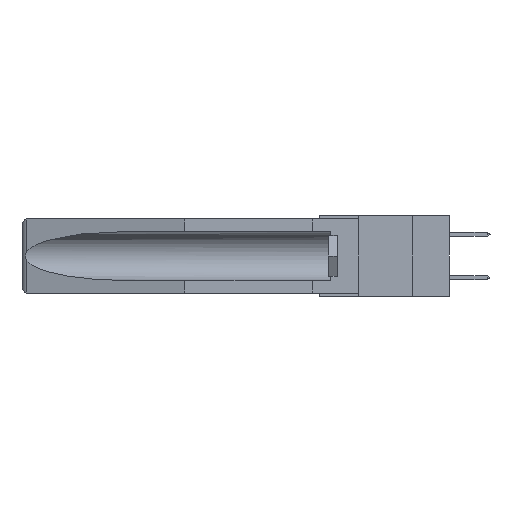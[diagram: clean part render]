
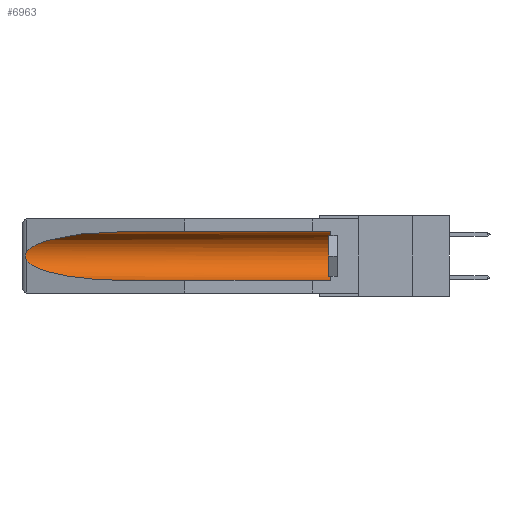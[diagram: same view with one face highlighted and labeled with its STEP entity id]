
A CAD part, left-side view. The second image highlights one B-rep face of the part: STEP entity #6963.
In plain terms, the highlighted cylindrical face has radius 2.857 mm (diameter 5.715 mm), a partial arc.
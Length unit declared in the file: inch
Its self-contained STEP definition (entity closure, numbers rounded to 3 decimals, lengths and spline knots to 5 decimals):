
#59 = VERTEX_POINT ( 'NONE', #10815 ) ;
#134 = DIRECTION ( 'NONE',  ( 0., 1., 0. ) ) ;
#174 = DIRECTION ( 'NONE',  ( 0., 1., 0. ) ) ;
#316 = FACE_OUTER_BOUND ( 'NONE', #22766, .T. ) ;
#932 = DIRECTION ( 'NONE',  ( 0., 0., 1. ) ) ;
#1498 = VERTEX_POINT ( 'NONE', #21890 ) ;
#1548 = CIRCLE ( 'NONE', #16449, 0.1125 ) ;
#3042 = LINE ( 'NONE', #25327, #4693 ) ;
#3285 = CARTESIAN_POINT ( 'NONE',  ( 0.26655, 1.53094, -0.18657 ) ) ;
#3318 = CARTESIAN_POINT ( 'NONE',  ( 0.25451, 1.48313, -0.24835 ) ) ;
#4693 = VECTOR ( 'NONE', #9252, 39.37008 ) ;
#4978 = CARTESIAN_POINT ( 'NONE',  ( 0.25451, 1.48313, -0.09465 ) ) ;
#6385 = DIRECTION ( 'NONE',  ( 0., -1., 0. ) ) ;
#6556 = CARTESIAN_POINT ( 'NONE',  ( 0.155, 1.07973, -0.284 ) ) ;
#6676 = AXIS2_PLACEMENT_3D ( 'NONE', #10290, #134, #32655 ) ;
#6963 = ADVANCED_FACE ( 'NONE', ( #316 ), #26231, .F. ) ;
#7636 = CARTESIAN_POINT ( 'NONE',  ( 0.26537, 1.52718, -0.14972 ) ) ;
#8374 = CARTESIAN_POINT ( 'NONE',  ( 0.2673, 1.53269, -0.17917 ) ) ;
#8610 = CARTESIAN_POINT ( 'NONE',  ( 0.26597, 1.5296, -0.19026 ) ) ;
#9143 = ORIENTED_EDGE ( 'NONE', *, *, #29280, .T. ) ;
#9252 = DIRECTION ( 'NONE',  ( 0., 1., 0. ) ) ;
#10238 = CARTESIAN_POINT ( 'NONE',  ( 0.21114, 1.30732, -0.059 ) ) ;
#10290 = CARTESIAN_POINT ( 'NONE',  ( 0.155, -0.30754, -0.1715 ) ) ;
#10815 = CARTESIAN_POINT ( 'NONE',  ( 0.26537, 1.52718, -0.14972 ) ) ;
#11395 = CARTESIAN_POINT ( 'NONE',  ( 0.155, 0.126, -0.059 ) ) ;
#11429 = CARTESIAN_POINT ( 'NONE',  ( 0.2675, 1.53308, -0.16763 ) ) ;
#11684 = CARTESIAN_POINT ( 'NONE',  ( 0.155, 1.07973, -0.284 ) ) ;
#13433 = ORIENTED_EDGE ( 'NONE', *, *, #33582, .T. ) ;
#15257 = EDGE_CURVE ( 'NONE', #30321, #20262, #20143, .T. ) ;
#15938 = CARTESIAN_POINT ( 'NONE',  ( 0.155, 0.126, -0.284 ) ) ;
#16397 = CARTESIAN_POINT ( 'NONE',  ( 0.26597, 1.52961, -0.15275 ) ) ;
#16449 = AXIS2_PLACEMENT_3D ( 'NONE', #19545, #6385, #932 ) ;
#16843 = CARTESIAN_POINT ( 'NONE',  ( 0.26654, 1.53092, -0.15636 ) ) ;
#18236 = CARTESIAN_POINT ( 'NONE',  ( 0.155, 1.07973, -0.059 ) ) ;
#19545 = CARTESIAN_POINT ( 'NONE',  ( 0.155, 0.126, -0.1715 ) ) ;
#20061 =( BOUNDED_CURVE ( )  B_SPLINE_CURVE ( 3, ( #27736, #3318, #29985, #11684 ),
 .UNSPECIFIED., .F., .F. ) 
 B_SPLINE_CURVE_WITH_KNOTS ( ( 4, 4 ),
 ( 0.1948, 1.5708 ),
 .UNSPECIFIED. ) 
 CURVE ( )  GEOMETRIC_REPRESENTATION_ITEM ( )  RATIONAL_B_SPLINE_CURVE ( ( 1., 0.848, 0.848, 1. ) ) 
 REPRESENTATION_ITEM ( '' )  );
#20143 = LINE ( 'NONE', #24149, #22635 ) ;
#20262 = VERTEX_POINT ( 'NONE', #25999 ) ;
#20986 = ORIENTED_EDGE ( 'NONE', *, *, #15257, .T. ) ;
#21890 = CARTESIAN_POINT ( 'NONE',  ( 0.26537, 1.52718, -0.19328 ) ) ;
#22635 = VECTOR ( 'NONE', #174, 39.37008 ) ;
#22766 = EDGE_LOOP ( 'NONE', ( #13433, #28427, #9143, #25375, #30337, #20986 ) ) ;
#24149 = CARTESIAN_POINT ( 'NONE',  ( 0.155, -0.30754, -0.059 ) ) ;
#24269 = EDGE_CURVE ( 'NONE', #25095, #30321, #1548, .T. ) ;
#24566 = CARTESIAN_POINT ( 'NONE',  ( 0.26537, 1.52718, -0.14972 ) ) ;
#25095 = VERTEX_POINT ( 'NONE', #15938 ) ;
#25191 =( BOUNDED_CURVE ( )  B_SPLINE_CURVE ( 3, ( #18236, #10238, #4978, #7636 ),
 .UNSPECIFIED., .F., .F. ) 
 B_SPLINE_CURVE_WITH_KNOTS ( ( 4, 4 ),
 ( 4.71239, 6.08839 ),
 .UNSPECIFIED. ) 
 CURVE ( )  GEOMETRIC_REPRESENTATION_ITEM ( )  RATIONAL_B_SPLINE_CURVE ( ( 1., 0.848, 0.848, 1. ) ) 
 REPRESENTATION_ITEM ( '' )  );
#25327 = CARTESIAN_POINT ( 'NONE',  ( 0.155, -0.30754, -0.284 ) ) ;
#25375 = ORIENTED_EDGE ( 'NONE', *, *, #26642, .F. ) ;
#25999 = CARTESIAN_POINT ( 'NONE',  ( 0.155, 1.07973, -0.059 ) ) ;
#26231 = CYLINDRICAL_SURFACE ( 'NONE', #6676, 0.1125 ) ;
#26642 = EDGE_CURVE ( 'NONE', #25095, #27997, #3042, .T. ) ;
#27014 = CARTESIAN_POINT ( 'NONE',  ( 0.26537, 1.52718, -0.19328 ) ) ;
#27359 = CARTESIAN_POINT ( 'NONE',  ( 0.2675, 1.53308, -0.17534 ) ) ;
#27478 = CARTESIAN_POINT ( 'NONE',  ( 0.2673, 1.5327, -0.16383 ) ) ;
#27736 = CARTESIAN_POINT ( 'NONE',  ( 0.26537, 1.52718, -0.19328 ) ) ;
#27997 = VERTEX_POINT ( 'NONE', #6556 ) ;
#28427 = ORIENTED_EDGE ( 'NONE', *, *, #30977, .T. ) ;
#29280 = EDGE_CURVE ( 'NONE', #1498, #27997, #20061, .T. ) ;
#29985 = CARTESIAN_POINT ( 'NONE',  ( 0.21114, 1.30732, -0.284 ) ) ;
#30321 = VERTEX_POINT ( 'NONE', #11395 ) ;
#30337 = ORIENTED_EDGE ( 'NONE', *, *, #24269, .T. ) ;
#30977 = EDGE_CURVE ( 'NONE', #59, #1498, #32511, .T. ) ;
#32511 = B_SPLINE_CURVE_WITH_KNOTS ( 'NONE', 3,
 ( #24566, #16397, #16843, #27478, #11429, #27359, #8374, #3285, #8610, #27014 ),
 .UNSPECIFIED., .F., .F.,
 ( 4, 2, 2, 2, 4 ),
 ( 0., 0.00029, 0.00058, 0.00087, 0.00117 ),
 .UNSPECIFIED. ) ;
#32655 = DIRECTION ( 'NONE',  ( 0., 0., 1. ) ) ;
#33582 = EDGE_CURVE ( 'NONE', #20262, #59, #25191, .T. ) ;
